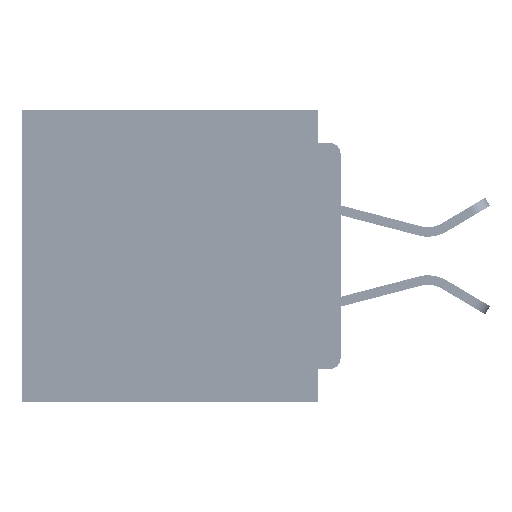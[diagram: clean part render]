
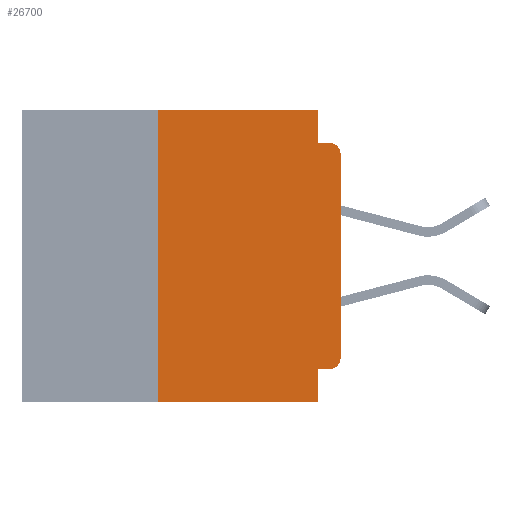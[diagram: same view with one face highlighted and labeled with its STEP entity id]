
A CAD part, left-side view. The second image highlights one B-rep face of the part: STEP entity #26700.
In plain terms, the highlighted planar face has unit normal (-1, 0, 0).
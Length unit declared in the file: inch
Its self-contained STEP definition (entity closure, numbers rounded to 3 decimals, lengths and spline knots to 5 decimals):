
#77 = DIRECTION ( 'NONE',  ( 1., 0., 0. ) ) ;
#520 = DIRECTION ( 'NONE',  ( 0., 0., 1. ) ) ;
#541 = AXIS2_PLACEMENT_3D ( 'NONE', #59461, #30921, #1989 ) ;
#741 = CIRCLE ( 'NONE', #55751, 0.015 ) ;
#1989 = DIRECTION ( 'NONE',  ( 0., 0., -1. ) ) ;
#2608 = ORIENTED_EDGE ( 'NONE', *, *, #46080, .T. ) ;
#3431 = CARTESIAN_POINT ( 'NONE',  ( 0., 0.031, -0.045 ) ) ;
#3732 = EDGE_CURVE ( 'NONE', #3819, #27145, #17076, .T. ) ;
#3819 = VERTEX_POINT ( 'NONE', #51762 ) ;
#7055 = ORIENTED_EDGE ( 'NONE', *, *, #18027, .F. ) ;
#8760 = CARTESIAN_POINT ( 'NONE',  ( 0., 0.437, 0. ) ) ;
#9016 = CARTESIAN_POINT ( 'NONE',  ( 0., 0., -0.045 ) ) ;
#9611 = VECTOR ( 'NONE', #60847, 39.37008 ) ;
#10370 = ORIENTED_EDGE ( 'NONE', *, *, #26019, .T. ) ;
#10443 = VERTEX_POINT ( 'NONE', #51916 ) ;
#10780 = EDGE_CURVE ( 'NONE', #10443, #38130, #49889, .T. ) ;
#11023 = LINE ( 'NONE', #8760, #22383 ) ;
#11651 = VECTOR ( 'NONE', #16751, 39.37008 ) ;
#11895 = CARTESIAN_POINT ( 'NONE',  ( 0., 0.031, -0.4 ) ) ;
#12812 = VECTOR ( 'NONE', #47664, 39.37008 ) ;
#13031 = CARTESIAN_POINT ( 'NONE',  ( 0., 0.031, 0. ) ) ;
#15181 = CARTESIAN_POINT ( 'NONE',  ( 0., 0., -0.355 ) ) ;
#15597 = VERTEX_POINT ( 'NONE', #37353 ) ;
#16751 = DIRECTION ( 'NONE',  ( 0., 0., -1. ) ) ;
#17076 = LINE ( 'NONE', #13031, #41036 ) ;
#17156 = VECTOR ( 'NONE', #520, 39.37008 ) ;
#18027 = EDGE_CURVE ( 'NONE', #31438, #3819, #11023, .T. ) ;
#19622 = CARTESIAN_POINT ( 'NONE',  ( 0., 0.015, -0.355 ) ) ;
#19669 = VECTOR ( 'NONE', #56539, 39.37008 ) ;
#21181 = CIRCLE ( 'NONE', #541, 0.015 ) ;
#22000 = EDGE_CURVE ( 'NONE', #35416, #38130, #45124, .T. ) ;
#22383 = VECTOR ( 'NONE', #47016, 39.37008 ) ;
#23275 = DIRECTION ( 'NONE',  ( -1., 0., 0. ) ) ;
#24286 = AXIS2_PLACEMENT_3D ( 'NONE', #29060, #77, #33900 ) ;
#24632 = FACE_OUTER_BOUND ( 'NONE', #30300, .T. ) ;
#25953 = CARTESIAN_POINT ( 'NONE',  ( 0., 0.25, -0.4 ) ) ;
#26019 = EDGE_CURVE ( 'NONE', #47163, #53843, #36692, .T. ) ;
#26412 = VECTOR ( 'NONE', #43883, 39.37008 ) ;
#26700 = ADVANCED_FACE ( 'NONE', ( #24632 ), #57622, .F. ) ;
#27105 = LINE ( 'NONE', #9016, #12812 ) ;
#27145 = VERTEX_POINT ( 'NONE', #3431 ) ;
#27525 = CARTESIAN_POINT ( 'NONE',  ( 0., 0., -0.34 ) ) ;
#29060 = CARTESIAN_POINT ( 'NONE',  ( 0., 0.437, 0. ) ) ;
#30300 = EDGE_LOOP ( 'NONE', ( #10370, #2608, #41414, #39344, #7055, #44068, #35954, #32495, #52141, #58180 ) ) ;
#30921 = DIRECTION ( 'NONE',  ( -1., 0., 0. ) ) ;
#31382 = LINE ( 'NONE', #34340, #17156 ) ;
#31438 = VERTEX_POINT ( 'NONE', #47657 ) ;
#32321 = DIRECTION ( 'NONE',  ( 0., 0., -1. ) ) ;
#32495 = ORIENTED_EDGE ( 'NONE', *, *, #10780, .F. ) ;
#33900 = DIRECTION ( 'NONE',  ( 0., 0., -1. ) ) ;
#34340 = CARTESIAN_POINT ( 'NONE',  ( 0., 0.25, -0.4 ) ) ;
#35416 = VERTEX_POINT ( 'NONE', #25953 ) ;
#35460 = CARTESIAN_POINT ( 'NONE',  ( 0., 0.031, -0.4 ) ) ;
#35954 = ORIENTED_EDGE ( 'NONE', *, *, #22000, .T. ) ;
#36692 = LINE ( 'NONE', #36948, #9611 ) ;
#36948 = CARTESIAN_POINT ( 'NONE',  ( 0., 0., 0. ) ) ;
#37353 = CARTESIAN_POINT ( 'NONE',  ( 0., 0.015, -0.045 ) ) ;
#38130 = VERTEX_POINT ( 'NONE', #35460 ) ;
#39344 = ORIENTED_EDGE ( 'NONE', *, *, #3732, .F. ) ;
#41036 = VECTOR ( 'NONE', #32321, 39.37008 ) ;
#41414 = ORIENTED_EDGE ( 'NONE', *, *, #46434, .F. ) ;
#43883 = DIRECTION ( 'NONE',  ( 0., 1., 0. ) ) ;
#44068 = ORIENTED_EDGE ( 'NONE', *, *, #50615, .F. ) ;
#45124 = LINE ( 'NONE', #47253, #19669 ) ;
#46080 = EDGE_CURVE ( 'NONE', #53843, #15597, #21181, .T. ) ;
#46434 = EDGE_CURVE ( 'NONE', #27145, #15597, #27105, .T. ) ;
#47016 = DIRECTION ( 'NONE',  ( 0., -1., 0. ) ) ;
#47163 = VERTEX_POINT ( 'NONE', #27525 ) ;
#47253 = CARTESIAN_POINT ( 'NONE',  ( 0., 0.437, -0.4 ) ) ;
#47657 = CARTESIAN_POINT ( 'NONE',  ( 0., 0.25, 0. ) ) ;
#47664 = DIRECTION ( 'NONE',  ( 0., -1., 0. ) ) ;
#47807 = EDGE_CURVE ( 'NONE', #56098, #47163, #741, .T. ) ;
#49889 = LINE ( 'NONE', #11895, #11651 ) ;
#50325 = LINE ( 'NONE', #15181, #26412 ) ;
#50615 = EDGE_CURVE ( 'NONE', #35416, #31438, #31382, .T. ) ;
#50685 = CARTESIAN_POINT ( 'NONE',  ( 0., 0., -0.06 ) ) ;
#51762 = CARTESIAN_POINT ( 'NONE',  ( 0., 0.031, 0. ) ) ;
#51866 = CARTESIAN_POINT ( 'NONE',  ( 0., 0.015, -0.34 ) ) ;
#51916 = CARTESIAN_POINT ( 'NONE',  ( 0., 0.031, -0.355 ) ) ;
#52141 = ORIENTED_EDGE ( 'NONE', *, *, #58776, .F. ) ;
#53843 = VERTEX_POINT ( 'NONE', #50685 ) ;
#55751 = AXIS2_PLACEMENT_3D ( 'NONE', #51866, #23275, #56605 ) ;
#56098 = VERTEX_POINT ( 'NONE', #19622 ) ;
#56539 = DIRECTION ( 'NONE',  ( 0., -1., 0. ) ) ;
#56605 = DIRECTION ( 'NONE',  ( 0., 0., -1. ) ) ;
#57622 = PLANE ( 'NONE',  #24286 ) ;
#58180 = ORIENTED_EDGE ( 'NONE', *, *, #47807, .T. ) ;
#58776 = EDGE_CURVE ( 'NONE', #56098, #10443, #50325, .T. ) ;
#59461 = CARTESIAN_POINT ( 'NONE',  ( 0., 0.015, -0.06 ) ) ;
#60847 = DIRECTION ( 'NONE',  ( 0., 0., 1. ) ) ;
